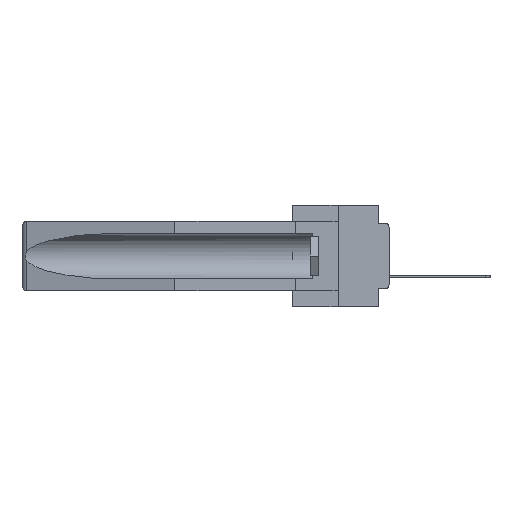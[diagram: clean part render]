
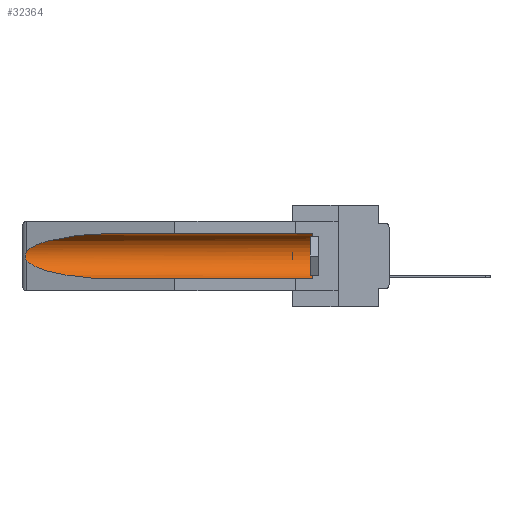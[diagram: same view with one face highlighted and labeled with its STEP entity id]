
A CAD part, left-side view. The second image highlights one B-rep face of the part: STEP entity #32364.
In plain terms, the highlighted cylindrical face has radius 2.857 mm (diameter 5.715 mm), a partial arc.
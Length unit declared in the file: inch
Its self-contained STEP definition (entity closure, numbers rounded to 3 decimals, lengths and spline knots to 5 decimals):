
#1015 = CARTESIAN_POINT ( 'NONE',  ( 0.26537, 1.52718, -0.14972 ) ) ;
#1031 = CIRCLE ( 'NONE', #40421, 0.1125 ) ;
#1444 = VECTOR ( 'NONE', #37311, 39.37008 ) ;
#1587 = VERTEX_POINT ( 'NONE', #29499 ) ;
#2011 = CARTESIAN_POINT ( 'NONE',  ( 0.155, 1.07973, -0.284 ) ) ;
#2577 = EDGE_CURVE ( 'NONE', #3160, #37941, #16992, .T. ) ;
#3160 = VERTEX_POINT ( 'NONE', #39113 ) ;
#3707 = ORIENTED_EDGE ( 'NONE', *, *, #12823, .T. ) ;
#5192 = CARTESIAN_POINT ( 'NONE',  ( 0.26537, 1.52718, -0.19328 ) ) ;
#5642 = LINE ( 'NONE', #14458, #1444 ) ;
#6064 = ORIENTED_EDGE ( 'NONE', *, *, #20810, .T. ) ;
#6632 = CARTESIAN_POINT ( 'NONE',  ( 0.21114, 1.30732, -0.284 ) ) ;
#7471 = ORIENTED_EDGE ( 'NONE', *, *, #36147, .T. ) ;
#7845 = DIRECTION ( 'NONE',  ( 0., 0., 1. ) ) ;
#8017 = CARTESIAN_POINT ( 'NONE',  ( 0.26537, 1.52718, -0.19328 ) ) ;
#8504 = DIRECTION ( 'NONE',  ( 0., -1., 0. ) ) ;
#8762 = VECTOR ( 'NONE', #29544, 39.37008 ) ;
#9055 = VERTEX_POINT ( 'NONE', #8017 ) ;
#10139 = ORIENTED_EDGE ( 'NONE', *, *, #25844, .T. ) ;
#12823 = EDGE_CURVE ( 'NONE', #9055, #37941, #24217, .T. ) ;
#13320 = CARTESIAN_POINT ( 'NONE',  ( 0.155, 1.07973, -0.059 ) ) ;
#13450 = B_SPLINE_CURVE_WITH_KNOTS ( 'NONE', 3,
 ( #20601, #21011, #30453, #18134, #33352, #15220, #36650, #36232, #30673, #5192 ),
 .UNSPECIFIED., .F., .F.,
 ( 4, 2, 2, 2, 4 ),
 ( 0., 0.00029, 0.00058, 0.00087, 0.00117 ),
 .UNSPECIFIED. ) ;
#14458 = CARTESIAN_POINT ( 'NONE',  ( 0.155, -0.30754, -0.059 ) ) ;
#14533 = VERTEX_POINT ( 'NONE', #22242 ) ;
#15220 = CARTESIAN_POINT ( 'NONE',  ( 0.2675, 1.53308, -0.17534 ) ) ;
#15255 = CARTESIAN_POINT ( 'NONE',  ( 0.155, 0.126, -0.1715 ) ) ;
#16992 = LINE ( 'NONE', #20298, #8762 ) ;
#17241 = EDGE_CURVE ( 'NONE', #32859, #9055, #13450, .T. ) ;
#18134 = CARTESIAN_POINT ( 'NONE',  ( 0.2673, 1.5327, -0.16383 ) ) ;
#18981 = CARTESIAN_POINT ( 'NONE',  ( 0.155, 1.07973, -0.284 ) ) ;
#19583 = CARTESIAN_POINT ( 'NONE',  ( 0.26537, 1.52718, -0.19328 ) ) ;
#20298 = CARTESIAN_POINT ( 'NONE',  ( 0.155, -0.30754, -0.284 ) ) ;
#20601 = CARTESIAN_POINT ( 'NONE',  ( 0.26537, 1.52718, -0.14972 ) ) ;
#20690 = AXIS2_PLACEMENT_3D ( 'NONE', #36028, #39093, #7845 ) ;
#20810 = EDGE_CURVE ( 'NONE', #14533, #1587, #5642, .T. ) ;
#21011 = CARTESIAN_POINT ( 'NONE',  ( 0.26597, 1.52961, -0.15275 ) ) ;
#21042 = DIRECTION ( 'NONE',  ( 0., 0., 1. ) ) ;
#21454 = ORIENTED_EDGE ( 'NONE', *, *, #2577, .F. ) ;
#21809 =( BOUNDED_CURVE ( )  B_SPLINE_CURVE ( 3, ( #13320, #28571, #25894, #1015 ),
 .UNSPECIFIED., .F., .F. ) 
 B_SPLINE_CURVE_WITH_KNOTS ( ( 4, 4 ),
 ( 4.71239, 6.08839 ),
 .UNSPECIFIED. ) 
 CURVE ( )  GEOMETRIC_REPRESENTATION_ITEM ( )  RATIONAL_B_SPLINE_CURVE ( ( 1., 0.848, 0.848, 1. ) ) 
 REPRESENTATION_ITEM ( '' )  );
#22242 = CARTESIAN_POINT ( 'NONE',  ( 0.155, 0.126, -0.059 ) ) ;
#24217 =( BOUNDED_CURVE ( )  B_SPLINE_CURVE ( 3, ( #19583, #34816, #6632, #18981 ),
 .UNSPECIFIED., .F., .F. ) 
 B_SPLINE_CURVE_WITH_KNOTS ( ( 4, 4 ),
 ( 0.1948, 1.5708 ),
 .UNSPECIFIED. ) 
 CURVE ( )  GEOMETRIC_REPRESENTATION_ITEM ( )  RATIONAL_B_SPLINE_CURVE ( ( 1., 0.848, 0.848, 1. ) ) 
 REPRESENTATION_ITEM ( '' )  );
#25844 = EDGE_CURVE ( 'NONE', #3160, #14533, #1031, .T. ) ;
#25894 = CARTESIAN_POINT ( 'NONE',  ( 0.25451, 1.48313, -0.09465 ) ) ;
#26552 = CYLINDRICAL_SURFACE ( 'NONE', #20690, 0.1125 ) ;
#28571 = CARTESIAN_POINT ( 'NONE',  ( 0.21114, 1.30732, -0.059 ) ) ;
#29499 = CARTESIAN_POINT ( 'NONE',  ( 0.155, 1.07973, -0.059 ) ) ;
#29544 = DIRECTION ( 'NONE',  ( 0., 1., 0. ) ) ;
#30227 = FACE_OUTER_BOUND ( 'NONE', #31414, .T. ) ;
#30453 = CARTESIAN_POINT ( 'NONE',  ( 0.26654, 1.53092, -0.15636 ) ) ;
#30673 = CARTESIAN_POINT ( 'NONE',  ( 0.26597, 1.5296, -0.19026 ) ) ;
#31414 = EDGE_LOOP ( 'NONE', ( #7471, #34570, #3707, #21454, #10139, #6064 ) ) ;
#32364 = ADVANCED_FACE ( 'NONE', ( #30227 ), #26552, .F. ) ;
#32859 = VERTEX_POINT ( 'NONE', #34244 ) ;
#33352 = CARTESIAN_POINT ( 'NONE',  ( 0.2675, 1.53308, -0.16763 ) ) ;
#34244 = CARTESIAN_POINT ( 'NONE',  ( 0.26537, 1.52718, -0.14972 ) ) ;
#34570 = ORIENTED_EDGE ( 'NONE', *, *, #17241, .T. ) ;
#34816 = CARTESIAN_POINT ( 'NONE',  ( 0.25451, 1.48313, -0.24835 ) ) ;
#36028 = CARTESIAN_POINT ( 'NONE',  ( 0.155, -0.30754, -0.1715 ) ) ;
#36147 = EDGE_CURVE ( 'NONE', #1587, #32859, #21809, .T. ) ;
#36232 = CARTESIAN_POINT ( 'NONE',  ( 0.26655, 1.53094, -0.18657 ) ) ;
#36650 = CARTESIAN_POINT ( 'NONE',  ( 0.2673, 1.53269, -0.17917 ) ) ;
#37311 = DIRECTION ( 'NONE',  ( 0., 1., 0. ) ) ;
#37941 = VERTEX_POINT ( 'NONE', #2011 ) ;
#39093 = DIRECTION ( 'NONE',  ( 0., 1., 0. ) ) ;
#39113 = CARTESIAN_POINT ( 'NONE',  ( 0.155, 0.126, -0.284 ) ) ;
#40421 = AXIS2_PLACEMENT_3D ( 'NONE', #15255, #8504, #21042 ) ;
